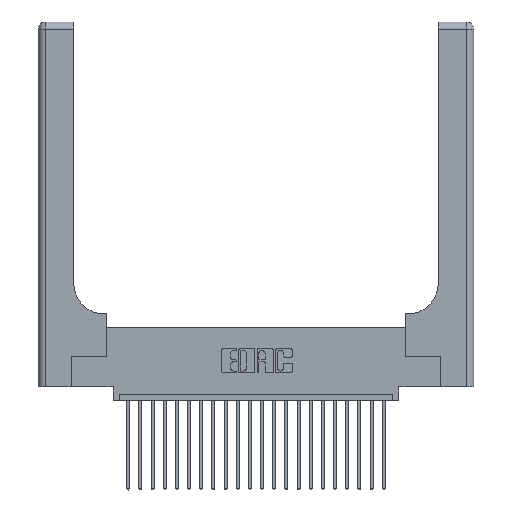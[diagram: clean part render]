
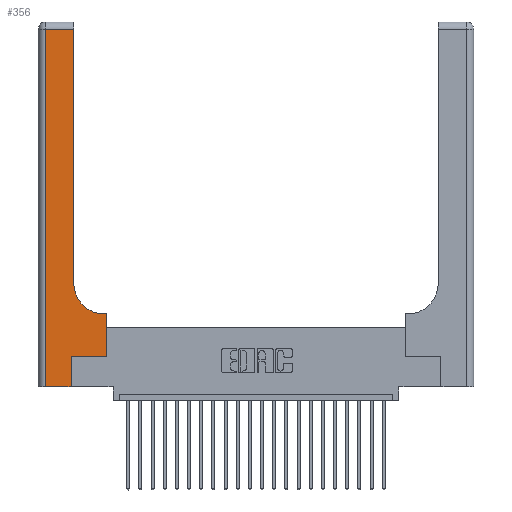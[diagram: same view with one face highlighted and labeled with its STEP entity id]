
A CAD part, top view. The second image highlights one B-rep face of the part: STEP entity #356.
In plain terms, the highlighted planar face has unit normal (0, 0, 1).
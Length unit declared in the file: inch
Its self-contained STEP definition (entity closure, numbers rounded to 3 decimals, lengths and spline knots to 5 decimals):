
#356 = ADVANCED_FACE ( 'NONE', ( #11349 ), #15172, .F. ) ;
#521 = DIRECTION ( 'NONE',  ( 1., 0., 0. ) ) ;
#683 = CARTESIAN_POINT ( 'NONE',  ( 0., 2.94, 0.37 ) ) ;
#740 = EDGE_CURVE ( 'NONE', #15598, #22691, #11326, .T. ) ;
#748 = EDGE_CURVE ( 'NONE', #18001, #22298, #7479, .T. ) ;
#938 = EDGE_CURVE ( 'NONE', #17129, #15598, #16694, .T. ) ;
#1014 = DIRECTION ( 'NONE',  ( 0., 1., 0. ) ) ;
#1246 = CARTESIAN_POINT ( 'NONE',  ( 0.2915, 2.94, 0.37 ) ) ;
#1294 = DIRECTION ( 'NONE',  ( 0., 1., 0. ) ) ;
#1482 = VERTEX_POINT ( 'NONE', #1246 ) ;
#1523 = CARTESIAN_POINT ( 'NONE',  ( 0.06, 0., 0.37 ) ) ;
#1793 = ORIENTED_EDGE ( 'NONE', *, *, #19845, .T. ) ;
#1812 = DIRECTION ( 'NONE',  ( 1., 0., 0. ) ) ;
#1828 = EDGE_CURVE ( 'NONE', #22691, #18001, #20988, .T. ) ;
#1970 = DIRECTION ( 'NONE',  ( 1., 0., 0. ) ) ;
#2942 = DIRECTION ( 'NONE',  ( -1., 0., 0. ) ) ;
#2968 = CARTESIAN_POINT ( 'NONE',  ( 0.06, 3., 0.37 ) ) ;
#2996 = ORIENTED_EDGE ( 'NONE', *, *, #4725, .T. ) ;
#3817 = ORIENTED_EDGE ( 'NONE', *, *, #10494, .T. ) ;
#3820 = VERTEX_POINT ( 'NONE', #13770 ) ;
#4692 = CARTESIAN_POINT ( 'NONE',  ( 0.5585, 0.25, 0.37 ) ) ;
#4725 = EDGE_CURVE ( 'NONE', #3820, #1482, #9252, .T. ) ;
#5388 = DIRECTION ( 'NONE',  ( 0., 0., -1. ) ) ;
#6265 = VECTOR ( 'NONE', #10647, 39.37008 ) ;
#6298 = VECTOR ( 'NONE', #521, 39.37008 ) ;
#6379 = DIRECTION ( 'NONE',  ( -1., 0., 0. ) ) ;
#6467 = ORIENTED_EDGE ( 'NONE', *, *, #938, .T. ) ;
#6937 = CARTESIAN_POINT ( 'NONE',  ( 0.2915, 3., 0.37 ) ) ;
#7040 = ORIENTED_EDGE ( 'NONE', *, *, #748, .T. ) ;
#7415 = CARTESIAN_POINT ( 'NONE',  ( 0.5585, 0.6, 0.37 ) ) ;
#7479 = LINE ( 'NONE', #21871, #9268 ) ;
#7842 = DIRECTION ( 'NONE',  ( -1., 0., 0. ) ) ;
#8197 = CARTESIAN_POINT ( 'NONE',  ( 0.269, 0.25, 0.37 ) ) ;
#8319 = LINE ( 'NONE', #2968, #6265 ) ;
#8956 = CARTESIAN_POINT ( 'NONE',  ( 0.5585, 0.25, 0.37 ) ) ;
#9121 = CARTESIAN_POINT ( 'NONE',  ( 0.5415, 0.6, 0.37 ) ) ;
#9160 = CARTESIAN_POINT ( 'NONE',  ( 0.5415, 0.85, 0.37 ) ) ;
#9252 = LINE ( 'NONE', #6937, #20856 ) ;
#9268 = VECTOR ( 'NONE', #2942, 39.37008 ) ;
#9292 = CARTESIAN_POINT ( 'NONE',  ( 0.06, 2.94, 0.37 ) ) ;
#9883 = CARTESIAN_POINT ( 'NONE',  ( 0.269, 0., 0.37 ) ) ;
#9926 = EDGE_CURVE ( 'NONE', #22298, #3820, #16350, .T. ) ;
#10494 = EDGE_CURVE ( 'NONE', #22375, #22811, #8319, .T. ) ;
#10647 = DIRECTION ( 'NONE',  ( 0., -1., 0. ) ) ;
#11326 = LINE ( 'NONE', #8197, #6298 ) ;
#11349 = FACE_OUTER_BOUND ( 'NONE', #19618, .T. ) ;
#13117 = CARTESIAN_POINT ( 'NONE',  ( 0., 3., 0.37 ) ) ;
#13770 = CARTESIAN_POINT ( 'NONE',  ( 0.2915, 0.85, 0.37 ) ) ;
#14762 = VECTOR ( 'NONE', #1294, 39.37008 ) ;
#15172 = PLANE ( 'NONE',  #21643 ) ;
#15598 = VERTEX_POINT ( 'NONE', #22922 ) ;
#16350 = CIRCLE ( 'NONE', #17807, 0.25 ) ;
#16694 = LINE ( 'NONE', #17749, #23551 ) ;
#16817 = ORIENTED_EDGE ( 'NONE', *, *, #9926, .T. ) ;
#17129 = VERTEX_POINT ( 'NONE', #9883 ) ;
#17522 = DIRECTION ( 'NONE',  ( 0., 1., 0. ) ) ;
#17749 = CARTESIAN_POINT ( 'NONE',  ( 0.269, 0., 0.37 ) ) ;
#17807 = AXIS2_PLACEMENT_3D ( 'NONE', #9160, #5388, #1812 ) ;
#18001 = VERTEX_POINT ( 'NONE', #7415 ) ;
#18312 = VECTOR ( 'NONE', #6379, 39.37008 ) ;
#18602 = LINE ( 'NONE', #683, #18312 ) ;
#18930 = LINE ( 'NONE', #21060, #23695 ) ;
#19326 = ORIENTED_EDGE ( 'NONE', *, *, #740, .T. ) ;
#19618 = EDGE_LOOP ( 'NONE', ( #2996, #1793, #3817, #20401, #6467, #19326, #23386, #7040, #16817 ) ) ;
#19845 = EDGE_CURVE ( 'NONE', #1482, #22375, #18602, .T. ) ;
#20401 = ORIENTED_EDGE ( 'NONE', *, *, #24362, .T. ) ;
#20594 = DIRECTION ( 'NONE',  ( 0., 0., -1. ) ) ;
#20856 = VECTOR ( 'NONE', #1014, 39.37008 ) ;
#20988 = LINE ( 'NONE', #8956, #14762 ) ;
#21060 = CARTESIAN_POINT ( 'NONE',  ( 0., 0., 0.37 ) ) ;
#21643 = AXIS2_PLACEMENT_3D ( 'NONE', #13117, #20594, #7842 ) ;
#21871 = CARTESIAN_POINT ( 'NONE',  ( 0.2915, 0.6, 0.37 ) ) ;
#22298 = VERTEX_POINT ( 'NONE', #9121 ) ;
#22375 = VERTEX_POINT ( 'NONE', #9292 ) ;
#22691 = VERTEX_POINT ( 'NONE', #4692 ) ;
#22811 = VERTEX_POINT ( 'NONE', #1523 ) ;
#22922 = CARTESIAN_POINT ( 'NONE',  ( 0.269, 0.25, 0.37 ) ) ;
#23386 = ORIENTED_EDGE ( 'NONE', *, *, #1828, .T. ) ;
#23551 = VECTOR ( 'NONE', #17522, 39.37008 ) ;
#23695 = VECTOR ( 'NONE', #1970, 39.37008 ) ;
#24362 = EDGE_CURVE ( 'NONE', #22811, #17129, #18930, .T. ) ;
